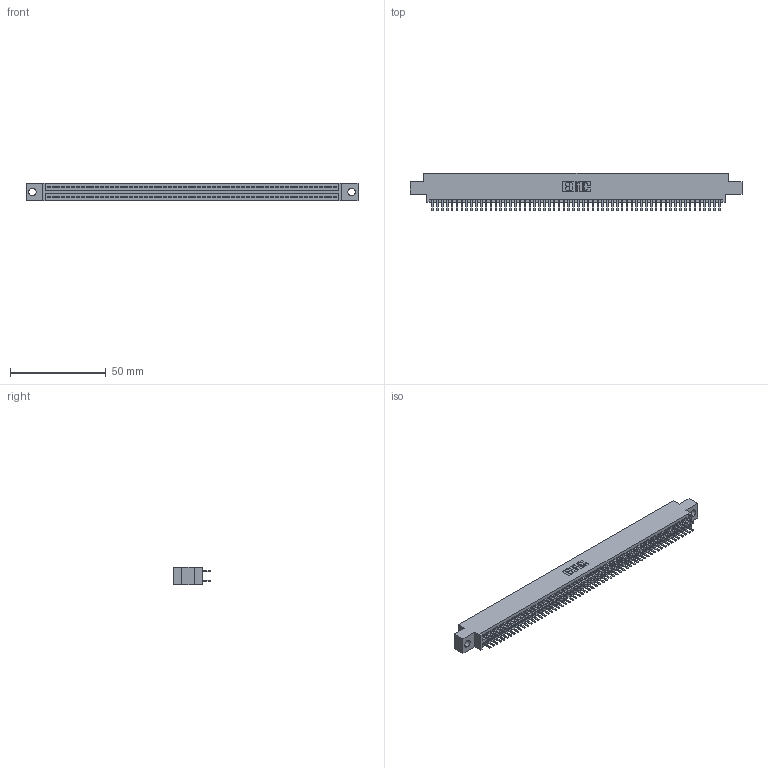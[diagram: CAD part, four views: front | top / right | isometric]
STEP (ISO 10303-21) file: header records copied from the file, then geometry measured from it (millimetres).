
FILE_DESCRIPTION (( 'STEP AP203' ), '1' );
FILE_NAME ('395-120-520-804.STEP', '2021-06-17T20:33:51', ( '' ), ( '' ), 'SwSTEP 2.0', 'SolidWorks 2020', '' );
FILE_SCHEMA (( 'CONFIG_CONTROL_DESIGN' ));
Length unit declared in the file: inch
Products named in the file (3): 345-292-001_345-293-120; 395-120-520-804; 345 Part_0.170 Offset - 0.156 Dia-TI
Assembly tree (121 placements, depth 2):
  395-120-520-804
    345 Part_0.170 Offset - 0.156 Dia-TI
    345-292-001_345-293-120  x120
Bounding box: 173.61 x 19.68 x 9.4 mm (x, y, z)
Volume: 16759.5 mm3; surface area: 25004.9 mm2
Topology: 121 solids, 121 shells, 6624 faces, 19229 edges, 12498 vertices
Faces by surface type: plane 4298, cylinder 2326
Entity records: 45319 total; most frequent: CARTESIAN_POINT 7598, ORIENTED_EDGE 7518, DIRECTION 6663, EDGE_CURVE 3759, VECTOR 3383, LINE 3383, VERTEX_POINT 2502, AXIS2_PLACEMENT_3D 1640
